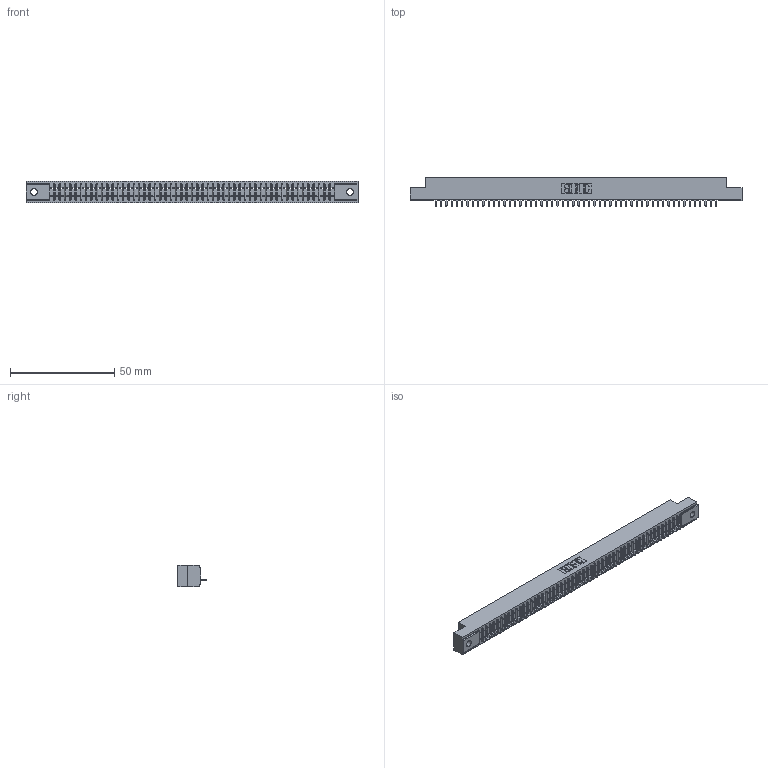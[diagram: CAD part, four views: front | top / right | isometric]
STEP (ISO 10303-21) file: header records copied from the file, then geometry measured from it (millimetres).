
FILE_DESCRIPTION (( 'STEP AP203' ), '1' );
FILE_NAME ('391-054-524-102.STEP', '2018-08-09T07:11:05', ( '' ), ( '' ), 'SwSTEP 2.0', 'SolidWorks 2016', '' );
FILE_SCHEMA (( 'CONFIG_CONTROL_DESIGN' ));
Length unit declared in the file: inch
Products named in the file (3): 341-292-001_341-292-124; 391-054-524-102; 341 Part_.128 (3.25) Dia Mounting Holes
Assembly tree (55 placements, depth 2):
  391-054-524-102
    341 Part_.128 (3.25) Dia Mounting Holes
    341-292-001_341-292-124  x54
Bounding box: 159.38 x 13.64 x 10.16 mm (x, y, z)
Volume: 11348.7 mm3; surface area: 17480.3 mm2
Topology: 55 solids, 55 shells, 4544 faces, 13114 edges, 8414 vertices
Faces by surface type: plane 2822, cylinder 1506, sphere 110, torus 106
Entity records: 62027 total; most frequent: CARTESIAN_POINT 10544, ORIENTED_EDGE 10532, DIRECTION 10168, EDGE_CURVE 5266, LINE 4268, VECTOR 4268, VERTEX_POINT 3326, AXIS2_PLACEMENT_3D 2950
